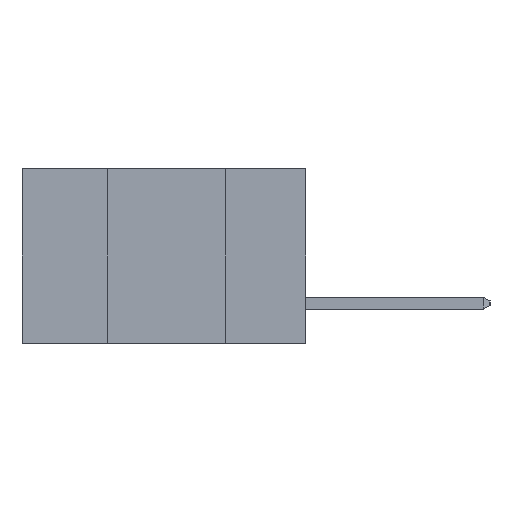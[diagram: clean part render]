
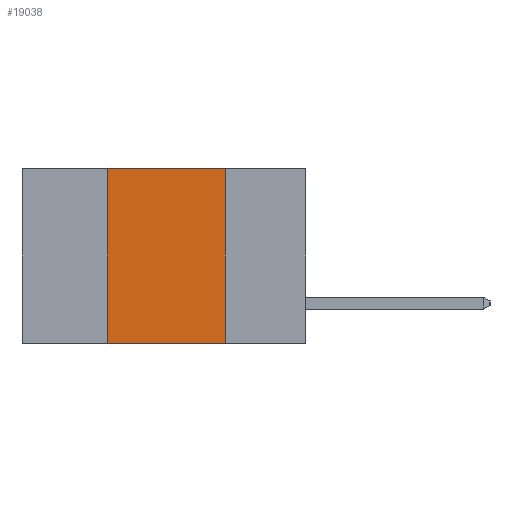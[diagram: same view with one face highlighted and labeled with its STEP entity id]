
A CAD part, left-side view. The second image highlights one B-rep face of the part: STEP entity #19038.
In plain terms, the highlighted planar face has unit normal (-1, 0, 0).
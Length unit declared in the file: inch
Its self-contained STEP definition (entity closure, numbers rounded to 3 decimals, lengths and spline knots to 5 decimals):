
#480 = DIRECTION ( 'NONE',  ( 0., 0., -1. ) ) ;
#841 = ORIENTED_EDGE ( 'NONE', *, *, #4786, .F. ) ;
#1176 = CARTESIAN_POINT ( 'NONE',  ( 0., 0.42, 0. ) ) ;
#2009 = EDGE_CURVE ( 'NONE', #5376, #16321, #15279, .T. ) ;
#2877 = ORIENTED_EDGE ( 'NONE', *, *, #2009, .F. ) ;
#3486 = DIRECTION ( 'NONE',  ( 0., 0., -1. ) ) ;
#4069 = LINE ( 'NONE', #20056, #19575 ) ;
#4089 = EDGE_LOOP ( 'NONE', ( #841, #16607, #2877, #8854 ) ) ;
#4786 = EDGE_CURVE ( 'NONE', #16277, #20606, #4069, .T. ) ;
#5376 = VERTEX_POINT ( 'NONE', #22974 ) ;
#5535 = CARTESIAN_POINT ( 'NONE',  ( 0., 0.17, -0.37 ) ) ;
#5860 = CARTESIAN_POINT ( 'NONE',  ( 0., 0.42, 0. ) ) ;
#5901 = LINE ( 'NONE', #12449, #20097 ) ;
#8706 = CARTESIAN_POINT ( 'NONE',  ( 0., 0.6, -0.37 ) ) ;
#8854 = ORIENTED_EDGE ( 'NONE', *, *, #22132, .T. ) ;
#9061 = FACE_OUTER_BOUND ( 'NONE', #4089, .T. ) ;
#10476 = DIRECTION ( 'NONE',  ( 0., 0., 1. ) ) ;
#10585 = PLANE ( 'NONE',  #17043 ) ;
#11633 = EDGE_CURVE ( 'NONE', #16321, #16277, #5901, .T. ) ;
#12371 = DIRECTION ( 'NONE',  ( 0., -1., 0. ) ) ;
#12449 = CARTESIAN_POINT ( 'NONE',  ( 0., 0.6, 0. ) ) ;
#12497 = DIRECTION ( 'NONE',  ( 1., 0., 0. ) ) ;
#15279 = LINE ( 'NONE', #1176, #24191 ) ;
#16277 = VERTEX_POINT ( 'NONE', #23024 ) ;
#16321 = VERTEX_POINT ( 'NONE', #5860 ) ;
#16500 = LINE ( 'NONE', #8706, #17107 ) ;
#16607 = ORIENTED_EDGE ( 'NONE', *, *, #11633, .F. ) ;
#17043 = AXIS2_PLACEMENT_3D ( 'NONE', #23861, #12497, #480 ) ;
#17107 = VECTOR ( 'NONE', #23958, 39.37008 ) ;
#19038 = ADVANCED_FACE ( 'NONE', ( #9061 ), #10585, .F. ) ;
#19575 = VECTOR ( 'NONE', #3486, 39.37008 ) ;
#20056 = CARTESIAN_POINT ( 'NONE',  ( 0., 0.17, 0. ) ) ;
#20097 = VECTOR ( 'NONE', #12371, 39.37008 ) ;
#20606 = VERTEX_POINT ( 'NONE', #5535 ) ;
#22132 = EDGE_CURVE ( 'NONE', #5376, #20606, #16500, .T. ) ;
#22974 = CARTESIAN_POINT ( 'NONE',  ( 0., 0.42, -0.37 ) ) ;
#23024 = CARTESIAN_POINT ( 'NONE',  ( 0., 0.17, 0. ) ) ;
#23861 = CARTESIAN_POINT ( 'NONE',  ( 0., 0.6, 0. ) ) ;
#23958 = DIRECTION ( 'NONE',  ( 0., -1., 0. ) ) ;
#24191 = VECTOR ( 'NONE', #10476, 39.37008 ) ;
